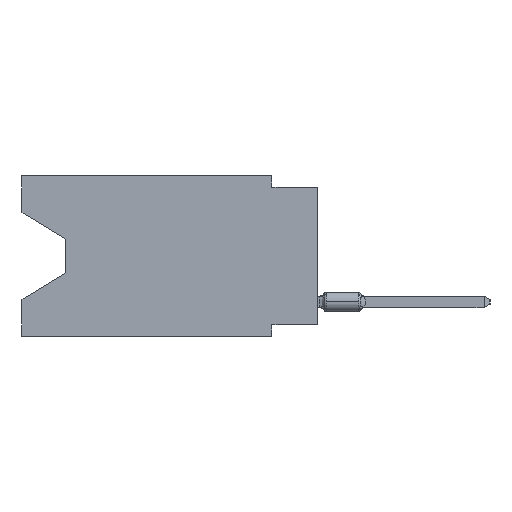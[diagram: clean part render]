
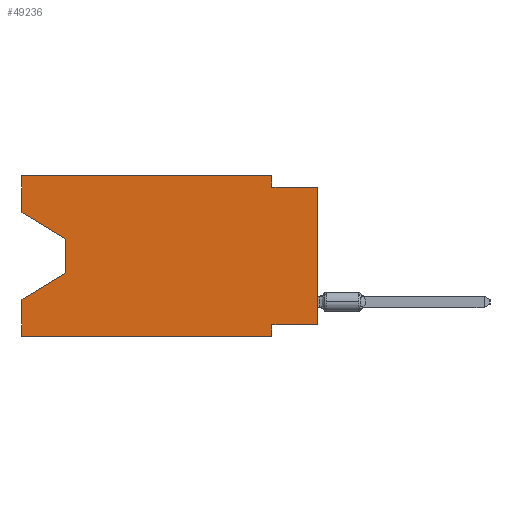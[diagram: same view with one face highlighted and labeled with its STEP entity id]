
A CAD part, left-side view. The second image highlights one B-rep face of the part: STEP entity #49236.
In plain terms, the highlighted planar face has unit normal (-1, 0, 0).
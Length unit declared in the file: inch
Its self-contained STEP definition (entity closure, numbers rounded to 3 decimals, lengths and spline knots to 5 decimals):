
#430 = LINE ( 'NONE', #27534, #4421 ) ;
#520 = CARTESIAN_POINT ( 'NONE',  ( 0., 0.1, -0.025 ) ) ;
#554 = VECTOR ( 'NONE', #24367, 39.37008 ) ;
#1193 = DIRECTION ( 'NONE',  ( 0., 0., 1. ) ) ;
#2630 = VECTOR ( 'NONE', #25831, 39.37008 ) ;
#3013 = DIRECTION ( 'NONE',  ( 0., 0., -1. ) ) ;
#3387 = VECTOR ( 'NONE', #12680, 39.37008 ) ;
#3456 = EDGE_CURVE ( 'NONE', #32958, #28886, #430, .T. ) ;
#4281 = VERTEX_POINT ( 'NONE', #36094 ) ;
#4421 = VECTOR ( 'NONE', #1193, 39.37008 ) ;
#4493 = LINE ( 'NONE', #47230, #3387 ) ;
#4642 = ORIENTED_EDGE ( 'NONE', *, *, #8157, .T. ) ;
#4921 = ORIENTED_EDGE ( 'NONE', *, *, #9359, .T. ) ;
#5977 = VERTEX_POINT ( 'NONE', #23229 ) ;
#7268 = EDGE_LOOP ( 'NONE', ( #14612, #4642, #34303, #30404, #4921, #31113, #13076, #28092, #19294, #7331, #35372, #28866 ) ) ;
#7331 = ORIENTED_EDGE ( 'NONE', *, *, #26601, .F. ) ;
#7481 = EDGE_CURVE ( 'NONE', #5977, #36980, #23477, .T. ) ;
#7517 = CARTESIAN_POINT ( 'NONE',  ( 0., 0., -0.325 ) ) ;
#7830 = DIRECTION ( 'NONE',  ( 0., 1., 0. ) ) ;
#8157 = EDGE_CURVE ( 'NONE', #36980, #38904, #23595, .T. ) ;
#9359 = EDGE_CURVE ( 'NONE', #17235, #40373, #39286, .T. ) ;
#9737 = CARTESIAN_POINT ( 'NONE',  ( 0., 0., -0.025 ) ) ;
#11873 = AXIS2_PLACEMENT_3D ( 'NONE', #30620, #19620, #3013 ) ;
#12680 = DIRECTION ( 'NONE',  ( 0., 0., -1. ) ) ;
#13076 = ORIENTED_EDGE ( 'NONE', *, *, #19574, .F. ) ;
#13106 = LINE ( 'NONE', #43555, #18581 ) ;
#13721 = VECTOR ( 'NONE', #31620, 39.37008 ) ;
#14578 = DIRECTION ( 'NONE',  ( 0., -0.855, -0.519 ) ) ;
#14612 = ORIENTED_EDGE ( 'NONE', *, *, #7481, .T. ) ;
#14784 = PLANE ( 'NONE',  #11873 ) ;
#14968 = DIRECTION ( 'NONE',  ( 0., 0., 1. ) ) ;
#15965 = EDGE_CURVE ( 'NONE', #17235, #37120, #47212, .T. ) ;
#17235 = VERTEX_POINT ( 'NONE', #30027 ) ;
#17790 = DIRECTION ( 'NONE',  ( 0., 0., -1. ) ) ;
#18581 = VECTOR ( 'NONE', #36374, 39.37008 ) ;
#18657 = CARTESIAN_POINT ( 'NONE',  ( 0., 0., -0.025 ) ) ;
#18787 = CARTESIAN_POINT ( 'NONE',  ( 0., 0.1, -0.325 ) ) ;
#19122 = LINE ( 'NONE', #27300, #29738 ) ;
#19294 = ORIENTED_EDGE ( 'NONE', *, *, #43665, .F. ) ;
#19574 = EDGE_CURVE ( 'NONE', #32958, #44537, #19122, .T. ) ;
#19620 = DIRECTION ( 'NONE',  ( 1., 0., 0. ) ) ;
#20985 = VERTEX_POINT ( 'NONE', #520 ) ;
#23229 = CARTESIAN_POINT ( 'NONE',  ( 0., 0.645, -0.08025 ) ) ;
#23477 = LINE ( 'NONE', #35004, #27563 ) ;
#23595 = LINE ( 'NONE', #28712, #554 ) ;
#24367 = DIRECTION ( 'NONE',  ( 0., 0., -1. ) ) ;
#24541 = CARTESIAN_POINT ( 'NONE',  ( 0., 0.55, -0.138 ) ) ;
#25831 = DIRECTION ( 'NONE',  ( 0., -1., 0. ) ) ;
#26481 = CARTESIAN_POINT ( 'NONE',  ( 0., 0.645, 0. ) ) ;
#26601 = EDGE_CURVE ( 'NONE', #4281, #20985, #37473, .T. ) ;
#26729 = EDGE_CURVE ( 'NONE', #5977, #42523, #37979, .T. ) ;
#27300 = CARTESIAN_POINT ( 'NONE',  ( 0., 0., -0.325 ) ) ;
#27534 = CARTESIAN_POINT ( 'NONE',  ( 0., 0., 0. ) ) ;
#27563 = VECTOR ( 'NONE', #14578, 39.37008 ) ;
#28092 = ORIENTED_EDGE ( 'NONE', *, *, #3456, .T. ) ;
#28712 = CARTESIAN_POINT ( 'NONE',  ( 0., 0.55, -0.138 ) ) ;
#28866 = ORIENTED_EDGE ( 'NONE', *, *, #26729, .F. ) ;
#28886 = VERTEX_POINT ( 'NONE', #9737 ) ;
#29108 = CARTESIAN_POINT ( 'NONE',  ( 0., 0.645, 0. ) ) ;
#29738 = VECTOR ( 'NONE', #7830, 39.37008 ) ;
#30027 = CARTESIAN_POINT ( 'NONE',  ( 0., 0.645, -0.35 ) ) ;
#30404 = ORIENTED_EDGE ( 'NONE', *, *, #15965, .F. ) ;
#30620 = CARTESIAN_POINT ( 'NONE',  ( 0., 0.645, 0. ) ) ;
#31113 = ORIENTED_EDGE ( 'NONE', *, *, #43058, .F. ) ;
#31205 = VECTOR ( 'NONE', #17790, 39.37008 ) ;
#31620 = DIRECTION ( 'NONE',  ( 0., -1., 0. ) ) ;
#31865 = DIRECTION ( 'NONE',  ( 0., 0., 1. ) ) ;
#32958 = VERTEX_POINT ( 'NONE', #7517 ) ;
#33185 = EDGE_CURVE ( 'NONE', #38904, #37120, #13106, .T. ) ;
#33432 = CARTESIAN_POINT ( 'NONE',  ( 0., 0.55, -0.212 ) ) ;
#33667 = VECTOR ( 'NONE', #14968, 39.37008 ) ;
#33841 = VECTOR ( 'NONE', #49093, 39.37008 ) ;
#34303 = ORIENTED_EDGE ( 'NONE', *, *, #33185, .T. ) ;
#35004 = CARTESIAN_POINT ( 'NONE',  ( 0., 0.645, -0.08025 ) ) ;
#35372 = ORIENTED_EDGE ( 'NONE', *, *, #47527, .F. ) ;
#35678 = CARTESIAN_POINT ( 'NONE',  ( 0., 0.645, 0. ) ) ;
#36094 = CARTESIAN_POINT ( 'NONE',  ( 0., 0.1, 0. ) ) ;
#36374 = DIRECTION ( 'NONE',  ( 0., 0.855, -0.519 ) ) ;
#36543 = VECTOR ( 'NONE', #31865, 39.37008 ) ;
#36980 = VERTEX_POINT ( 'NONE', #24541 ) ;
#37120 = VERTEX_POINT ( 'NONE', #41391 ) ;
#37473 = LINE ( 'NONE', #48513, #31205 ) ;
#37979 = LINE ( 'NONE', #26481, #33667 ) ;
#38904 = VERTEX_POINT ( 'NONE', #33432 ) ;
#39281 = CARTESIAN_POINT ( 'NONE',  ( 0., 0.1, -0.35 ) ) ;
#39286 = LINE ( 'NONE', #43638, #13721 ) ;
#40373 = VERTEX_POINT ( 'NONE', #39281 ) ;
#41170 = LINE ( 'NONE', #18657, #2630 ) ;
#41391 = CARTESIAN_POINT ( 'NONE',  ( 0., 0.645, -0.26975 ) ) ;
#42523 = VERTEX_POINT ( 'NONE', #46524 ) ;
#43058 = EDGE_CURVE ( 'NONE', #44537, #40373, #4493, .T. ) ;
#43555 = CARTESIAN_POINT ( 'NONE',  ( 0., 0.55, -0.212 ) ) ;
#43638 = CARTESIAN_POINT ( 'NONE',  ( 0., 0.645, -0.35 ) ) ;
#43665 = EDGE_CURVE ( 'NONE', #20985, #28886, #41170, .T. ) ;
#44537 = VERTEX_POINT ( 'NONE', #18787 ) ;
#46524 = CARTESIAN_POINT ( 'NONE',  ( 0., 0.645, 0. ) ) ;
#47212 = LINE ( 'NONE', #35678, #36543 ) ;
#47230 = CARTESIAN_POINT ( 'NONE',  ( 0., 0.1, -0.35 ) ) ;
#47527 = EDGE_CURVE ( 'NONE', #42523, #4281, #48565, .T. ) ;
#48513 = CARTESIAN_POINT ( 'NONE',  ( 0., 0.1, 0. ) ) ;
#48565 = LINE ( 'NONE', #29108, #33841 ) ;
#49093 = DIRECTION ( 'NONE',  ( 0., -1., 0. ) ) ;
#49236 = ADVANCED_FACE ( 'NONE', ( #49868 ), #14784, .F. ) ;
#49868 = FACE_OUTER_BOUND ( 'NONE', #7268, .T. ) ;
